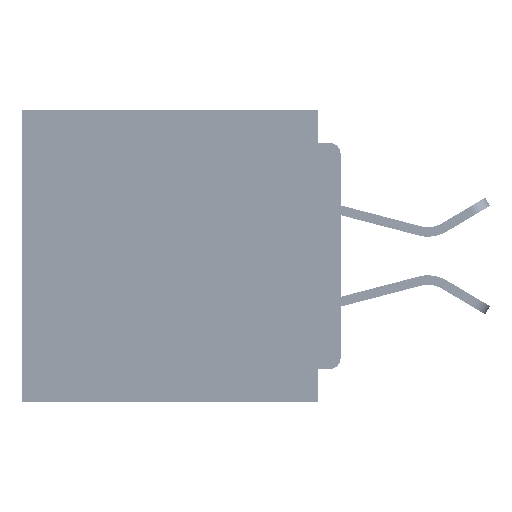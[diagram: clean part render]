
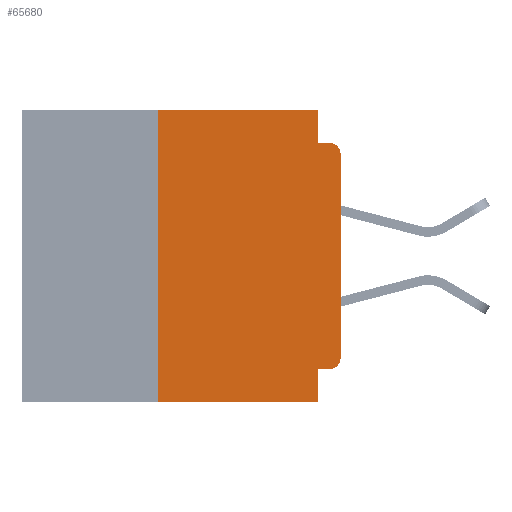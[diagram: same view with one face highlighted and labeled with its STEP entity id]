
A CAD part, left-side view. The second image highlights one B-rep face of the part: STEP entity #65680.
In plain terms, the highlighted planar face has unit normal (-1, 0, 0).
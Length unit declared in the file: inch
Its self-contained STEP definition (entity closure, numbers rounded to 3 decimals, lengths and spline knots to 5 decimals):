
#728 = CARTESIAN_POINT ( 'NONE',  ( 0., 0.015, -0.045 ) ) ;
#1220 = ORIENTED_EDGE ( 'NONE', *, *, #35451, .F. ) ;
#2118 = CARTESIAN_POINT ( 'NONE',  ( 0., 0.031, 0. ) ) ;
#2322 = DIRECTION ( 'NONE',  ( 0., 0., -1. ) ) ;
#3742 = CARTESIAN_POINT ( 'NONE',  ( 0., 0.437, 0. ) ) ;
#3997 = CIRCLE ( 'NONE', #17540, 0.015 ) ;
#5225 = ORIENTED_EDGE ( 'NONE', *, *, #63626, .T. ) ;
#5900 = EDGE_CURVE ( 'NONE', #24670, #13205, #21100, .T. ) ;
#6139 = EDGE_CURVE ( 'NONE', #22991, #30269, #34479, .T. ) ;
#7356 = LINE ( 'NONE', #69522, #19949 ) ;
#7488 = EDGE_CURVE ( 'NONE', #67994, #22991, #3997, .T. ) ;
#7685 = CARTESIAN_POINT ( 'NONE',  ( 0., 0.015, -0.34 ) ) ;
#7972 = ORIENTED_EDGE ( 'NONE', *, *, #5900, .F. ) ;
#8009 = DIRECTION ( 'NONE',  ( 0., 0., -1. ) ) ;
#8974 = PLANE ( 'NONE',  #44805 ) ;
#12481 = VERTEX_POINT ( 'NONE', #728 ) ;
#12551 = DIRECTION ( 'NONE',  ( 0., 0., 1. ) ) ;
#13078 = DIRECTION ( 'NONE',  ( 0., 0., -1. ) ) ;
#13205 = VERTEX_POINT ( 'NONE', #34038 ) ;
#15109 = ORIENTED_EDGE ( 'NONE', *, *, #7488, .T. ) ;
#15309 = EDGE_CURVE ( 'NONE', #54116, #24670, #25868, .T. ) ;
#16661 = DIRECTION ( 'NONE',  ( 0., -1., 0. ) ) ;
#17540 = AXIS2_PLACEMENT_3D ( 'NONE', #7685, #45278, #13078 ) ;
#17907 = VECTOR ( 'NONE', #8009, 39.37008 ) ;
#18267 = VERTEX_POINT ( 'NONE', #64989 ) ;
#19123 = VECTOR ( 'NONE', #66581, 39.37008 ) ;
#19949 = VECTOR ( 'NONE', #64130, 39.37008 ) ;
#19989 = DIRECTION ( 'NONE',  ( 1., 0., 0. ) ) ;
#20962 = CARTESIAN_POINT ( 'NONE',  ( 0., 0.25, -0.4 ) ) ;
#21100 = LINE ( 'NONE', #48071, #48013 ) ;
#22948 = ORIENTED_EDGE ( 'NONE', *, *, #6139, .T. ) ;
#22991 = VERTEX_POINT ( 'NONE', #35501 ) ;
#23494 = CARTESIAN_POINT ( 'NONE',  ( 0., 0., -0.06 ) ) ;
#24189 = VECTOR ( 'NONE', #69358, 39.37008 ) ;
#24430 = EDGE_LOOP ( 'NONE', ( #22948, #5225, #54030, #39107, #7972, #33455, #62645, #1220, #32040, #15109 ) ) ;
#24670 = VERTEX_POINT ( 'NONE', #50640 ) ;
#25868 = LINE ( 'NONE', #20962, #24189 ) ;
#27054 = CARTESIAN_POINT ( 'NONE',  ( 0., 0.031, -0.355 ) ) ;
#28270 = CARTESIAN_POINT ( 'NONE',  ( 0., 0.015, -0.355 ) ) ;
#29685 = EDGE_CURVE ( 'NONE', #13205, #18267, #62026, .T. ) ;
#30269 = VERTEX_POINT ( 'NONE', #23494 ) ;
#30521 = CARTESIAN_POINT ( 'NONE',  ( 0., 0.25, -0.4 ) ) ;
#31266 = EDGE_CURVE ( 'NONE', #54116, #62329, #62631, .T. ) ;
#31570 = AXIS2_PLACEMENT_3D ( 'NONE', #66787, #34541, #2322 ) ;
#32040 = ORIENTED_EDGE ( 'NONE', *, *, #50746, .F. ) ;
#32804 = VECTOR ( 'NONE', #12551, 39.37008 ) ;
#33430 = CIRCLE ( 'NONE', #31570, 0.015 ) ;
#33455 = ORIENTED_EDGE ( 'NONE', *, *, #15309, .F. ) ;
#34001 = VECTOR ( 'NONE', #16661, 39.37008 ) ;
#34038 = CARTESIAN_POINT ( 'NONE',  ( 0., 0.031, 0. ) ) ;
#34479 = LINE ( 'NONE', #44750, #32804 ) ;
#34541 = DIRECTION ( 'NONE',  ( -1., 0., 0. ) ) ;
#34999 = DIRECTION ( 'NONE',  ( 0., -1., 0. ) ) ;
#35451 = EDGE_CURVE ( 'NONE', #62000, #62329, #44833, .T. ) ;
#35501 = CARTESIAN_POINT ( 'NONE',  ( 0., 0., -0.34 ) ) ;
#37219 = DIRECTION ( 'NONE',  ( 0., -1., 0. ) ) ;
#39107 = ORIENTED_EDGE ( 'NONE', *, *, #29685, .F. ) ;
#41095 = LINE ( 'NONE', #61874, #57105 ) ;
#44750 = CARTESIAN_POINT ( 'NONE',  ( 0., 0., 0. ) ) ;
#44805 = AXIS2_PLACEMENT_3D ( 'NONE', #3742, #19989, #57599 ) ;
#44833 = LINE ( 'NONE', #45602, #17907 ) ;
#45278 = DIRECTION ( 'NONE',  ( -1., 0., 0. ) ) ;
#45602 = CARTESIAN_POINT ( 'NONE',  ( 0., 0.031, -0.4 ) ) ;
#48013 = VECTOR ( 'NONE', #37219, 39.37008 ) ;
#48071 = CARTESIAN_POINT ( 'NONE',  ( 0., 0.437, 0. ) ) ;
#48883 = CARTESIAN_POINT ( 'NONE',  ( 0., 0.437, -0.4 ) ) ;
#50640 = CARTESIAN_POINT ( 'NONE',  ( 0., 0.25, 0. ) ) ;
#50746 = EDGE_CURVE ( 'NONE', #67994, #62000, #7356, .T. ) ;
#51446 = CARTESIAN_POINT ( 'NONE',  ( 0., 0.031, -0.4 ) ) ;
#54030 = ORIENTED_EDGE ( 'NONE', *, *, #65582, .F. ) ;
#54116 = VERTEX_POINT ( 'NONE', #30521 ) ;
#57105 = VECTOR ( 'NONE', #34999, 39.37008 ) ;
#57599 = DIRECTION ( 'NONE',  ( 0., 0., -1. ) ) ;
#61874 = CARTESIAN_POINT ( 'NONE',  ( 0., 0., -0.045 ) ) ;
#62000 = VERTEX_POINT ( 'NONE', #27054 ) ;
#62026 = LINE ( 'NONE', #2118, #19123 ) ;
#62329 = VERTEX_POINT ( 'NONE', #51446 ) ;
#62631 = LINE ( 'NONE', #48883, #34001 ) ;
#62645 = ORIENTED_EDGE ( 'NONE', *, *, #31266, .T. ) ;
#62970 = FACE_OUTER_BOUND ( 'NONE', #24430, .T. ) ;
#63626 = EDGE_CURVE ( 'NONE', #30269, #12481, #33430, .T. ) ;
#64130 = DIRECTION ( 'NONE',  ( 0., 1., 0. ) ) ;
#64989 = CARTESIAN_POINT ( 'NONE',  ( 0., 0.031, -0.045 ) ) ;
#65582 = EDGE_CURVE ( 'NONE', #18267, #12481, #41095, .T. ) ;
#65680 = ADVANCED_FACE ( 'NONE', ( #62970 ), #8974, .F. ) ;
#66581 = DIRECTION ( 'NONE',  ( 0., 0., -1. ) ) ;
#66787 = CARTESIAN_POINT ( 'NONE',  ( 0., 0.015, -0.06 ) ) ;
#67994 = VERTEX_POINT ( 'NONE', #28270 ) ;
#69358 = DIRECTION ( 'NONE',  ( 0., 0., 1. ) ) ;
#69522 = CARTESIAN_POINT ( 'NONE',  ( 0., 0., -0.355 ) ) ;
